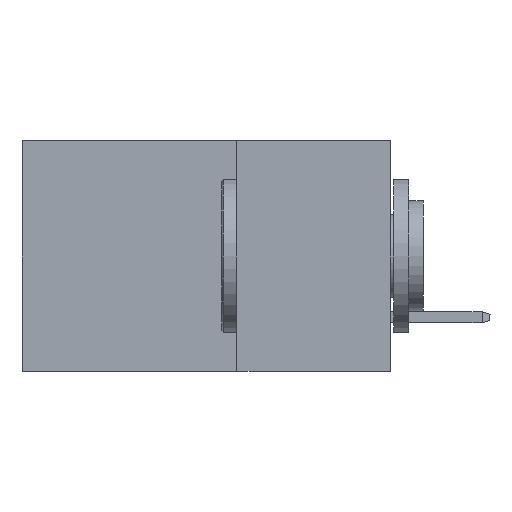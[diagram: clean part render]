
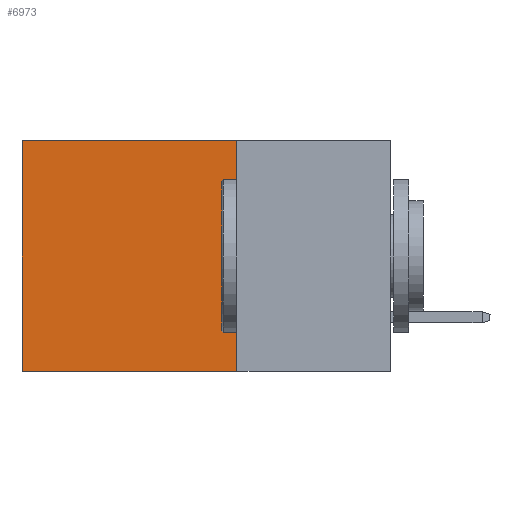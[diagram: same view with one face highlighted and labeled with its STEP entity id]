
A CAD part, left-side view. The second image highlights one B-rep face of the part: STEP entity #6973.
In plain terms, the highlighted planar face has unit normal (-1, 0, 0).
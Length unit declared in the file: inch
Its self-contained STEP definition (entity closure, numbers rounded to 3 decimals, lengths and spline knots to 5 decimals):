
#196 = ORIENTED_EDGE ( 'NONE', *, *, #10674, .F. ) ;
#258 = LINE ( 'NONE', #2984, #14006 ) ;
#357 = DIRECTION ( 'NONE',  ( 0., 0., -1. ) ) ;
#895 = CARTESIAN_POINT ( 'NONE',  ( 0.2875, 0.25, 0. ) ) ;
#1595 = EDGE_LOOP ( 'NONE', ( #11020, #11537, #196, #5464 ) ) ;
#2984 = CARTESIAN_POINT ( 'NONE',  ( 0.2875, 0.6, -0.375 ) ) ;
#4215 = CARTESIAN_POINT ( 'NONE',  ( 0.2875, 0.6, 0. ) ) ;
#4556 = VECTOR ( 'NONE', #14465, 39.37008 ) ;
#4937 = EDGE_CURVE ( 'NONE', #6722, #11442, #258, .T. ) ;
#5464 = ORIENTED_EDGE ( 'NONE', *, *, #13830, .T. ) ;
#6492 = CARTESIAN_POINT ( 'NONE',  ( 0.2875, 0.25, -0.375 ) ) ;
#6722 = VERTEX_POINT ( 'NONE', #4215 ) ;
#6873 = DIRECTION ( 'NONE',  ( 0., 1., 0. ) ) ;
#6973 = ADVANCED_FACE ( 'NONE', ( #14681 ), #14975, .F. ) ;
#6984 = CARTESIAN_POINT ( 'NONE',  ( 0.2875, 0.25, -0.375 ) ) ;
#7044 = CARTESIAN_POINT ( 'NONE',  ( 0.2875, 0.25, -0.375 ) ) ;
#7459 = LINE ( 'NONE', #7044, #14163 ) ;
#7795 = LINE ( 'NONE', #6984, #4556 ) ;
#7872 = LINE ( 'NONE', #895, #9999 ) ;
#8551 = CARTESIAN_POINT ( 'NONE',  ( 0.2875, 0.25, 0. ) ) ;
#8807 = EDGE_CURVE ( 'NONE', #11318, #11442, #7459, .T. ) ;
#9999 = VECTOR ( 'NONE', #6873, 39.37008 ) ;
#10204 = DIRECTION ( 'NONE',  ( 0., 0., -1. ) ) ;
#10674 = EDGE_CURVE ( 'NONE', #13299, #11318, #7795, .T. ) ;
#10762 = DIRECTION ( 'NONE',  ( 0., 1., 0. ) ) ;
#11020 = ORIENTED_EDGE ( 'NONE', *, *, #4937, .T. ) ;
#11318 = VERTEX_POINT ( 'NONE', #12815 ) ;
#11442 = VERTEX_POINT ( 'NONE', #14651 ) ;
#11537 = ORIENTED_EDGE ( 'NONE', *, *, #8807, .F. ) ;
#12815 = CARTESIAN_POINT ( 'NONE',  ( 0.2875, 0.25, -0.375 ) ) ;
#13299 = VERTEX_POINT ( 'NONE', #8551 ) ;
#13830 = EDGE_CURVE ( 'NONE', #13299, #6722, #7872, .T. ) ;
#13910 = DIRECTION ( 'NONE',  ( 1., 0., 0. ) ) ;
#14006 = VECTOR ( 'NONE', #10204, 39.37008 ) ;
#14163 = VECTOR ( 'NONE', #10762, 39.37008 ) ;
#14465 = DIRECTION ( 'NONE',  ( 0., 0., -1. ) ) ;
#14651 = CARTESIAN_POINT ( 'NONE',  ( 0.2875, 0.6, -0.375 ) ) ;
#14681 = FACE_OUTER_BOUND ( 'NONE', #1595, .T. ) ;
#14876 = AXIS2_PLACEMENT_3D ( 'NONE', #6492, #13910, #357 ) ;
#14975 = PLANE ( 'NONE',  #14876 ) ;
